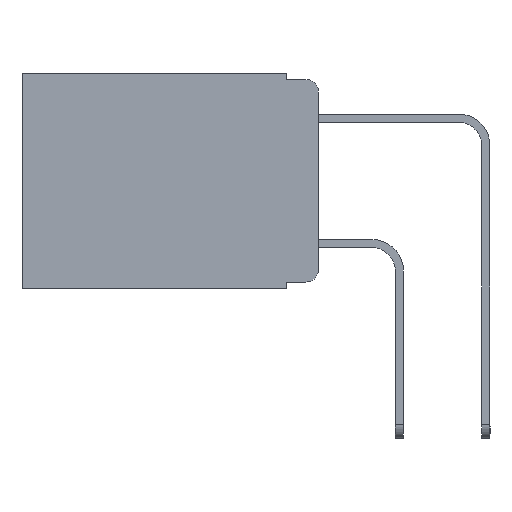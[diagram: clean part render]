
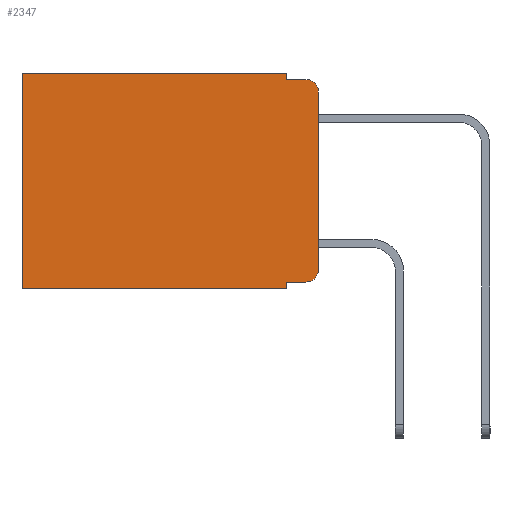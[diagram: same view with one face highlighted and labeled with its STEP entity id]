
A CAD part, left-side view. The second image highlights one B-rep face of the part: STEP entity #2347.
In plain terms, the highlighted planar face has unit normal (-1, 0, 0).
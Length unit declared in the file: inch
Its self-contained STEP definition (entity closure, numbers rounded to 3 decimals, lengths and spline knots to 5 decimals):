
#246 = EDGE_CURVE ( 'NONE', #7713, #7204, #11973, .T. ) ;
#724 = EDGE_CURVE ( 'NONE', #7204, #9671, #5408, .T. ) ;
#1034 = DIRECTION ( 'NONE',  ( 0., 0., -1. ) ) ;
#1077 = DIRECTION ( 'NONE',  ( -1., 0., 0. ) ) ;
#1807 = CARTESIAN_POINT ( 'NONE',  ( 0.298, 0.051, -0.343 ) ) ;
#1975 = VECTOR ( 'NONE', #14426, 39.37008 ) ;
#1977 = VECTOR ( 'NONE', #2763, 39.37008 ) ;
#2004 = ORIENTED_EDGE ( 'NONE', *, *, #11265, .T. ) ;
#2230 = DIRECTION ( 'NONE',  ( 0., 1., 0. ) ) ;
#2259 = CARTESIAN_POINT ( 'NONE',  ( 0.298, 0.051, 0. ) ) ;
#2347 = ADVANCED_FACE ( 'NONE', ( #16004 ), #14722, .F. ) ;
#2424 = LINE ( 'NONE', #2259, #12015 ) ;
#2763 = DIRECTION ( 'NONE',  ( 0., -1., 0. ) ) ;
#3219 = VERTEX_POINT ( 'NONE', #10655 ) ;
#3571 = ORIENTED_EDGE ( 'NONE', *, *, #6054, .T. ) ;
#3984 = CIRCLE ( 'NONE', #5084, 0.02 ) ;
#4034 = VECTOR ( 'NONE', #10815, 39.37008 ) ;
#4037 = VERTEX_POINT ( 'NONE', #16768 ) ;
#4116 = EDGE_CURVE ( 'NONE', #7650, #8345, #5388, .T. ) ;
#4186 = CARTESIAN_POINT ( 'NONE',  ( 0.298, 0., 0. ) ) ;
#4478 = CARTESIAN_POINT ( 'NONE',  ( 0.298, 0.02, -0.313 ) ) ;
#5084 = AXIS2_PLACEMENT_3D ( 'NONE', #5163, #1077, #13001 ) ;
#5163 = CARTESIAN_POINT ( 'NONE',  ( 0.298, 0.02, -0.03 ) ) ;
#5388 = LINE ( 'NONE', #6850, #5548 ) ;
#5408 = LINE ( 'NONE', #6866, #4034 ) ;
#5415 = CARTESIAN_POINT ( 'NONE',  ( 0.298, 0.02, -0.01 ) ) ;
#5548 = VECTOR ( 'NONE', #5563, 39.37008 ) ;
#5563 = DIRECTION ( 'NONE',  ( 0., 1., 0. ) ) ;
#5756 = EDGE_CURVE ( 'NONE', #16149, #7650, #2424, .T. ) ;
#5963 = LINE ( 'NONE', #14050, #16222 ) ;
#6054 = EDGE_CURVE ( 'NONE', #15632, #8345, #16400, .T. ) ;
#6850 = CARTESIAN_POINT ( 'NONE',  ( 0.298, 0., -0.343 ) ) ;
#6866 = CARTESIAN_POINT ( 'NONE',  ( 0.298, 0.051, -0.01 ) ) ;
#7204 = VERTEX_POINT ( 'NONE', #9839 ) ;
#7392 = DIRECTION ( 'NONE',  ( 0., 0., -1. ) ) ;
#7650 = VERTEX_POINT ( 'NONE', #1807 ) ;
#7713 = VERTEX_POINT ( 'NONE', #15015 ) ;
#7730 = CARTESIAN_POINT ( 'NONE',  ( 0.298, 0., 0. ) ) ;
#7798 = EDGE_CURVE ( 'NONE', #7713, #15632, #5963, .T. ) ;
#8127 = VECTOR ( 'NONE', #7392, 39.37008 ) ;
#8345 = VERTEX_POINT ( 'NONE', #14203 ) ;
#8360 = DIRECTION ( 'NONE',  ( 0., 0., -1. ) ) ;
#8661 = ORIENTED_EDGE ( 'NONE', *, *, #246, .F. ) ;
#9184 = DIRECTION ( 'NONE',  ( 1., 0., 0. ) ) ;
#9462 = ORIENTED_EDGE ( 'NONE', *, *, #724, .F. ) ;
#9671 = VERTEX_POINT ( 'NONE', #5415 ) ;
#9743 = DIRECTION ( 'NONE',  ( 0., 0., -1. ) ) ;
#9839 = CARTESIAN_POINT ( 'NONE',  ( 0.298, 0.051, -0.01 ) ) ;
#10168 = AXIS2_PLACEMENT_3D ( 'NONE', #4186, #9184, #10467 ) ;
#10467 = DIRECTION ( 'NONE',  ( 0., 0., -1. ) ) ;
#10603 = EDGE_CURVE ( 'NONE', #16149, #4037, #13464, .T. ) ;
#10655 = CARTESIAN_POINT ( 'NONE',  ( 0.298, 0., -0.03 ) ) ;
#10780 = CARTESIAN_POINT ( 'NONE',  ( 0.298, 0.051, -0.333 ) ) ;
#10815 = DIRECTION ( 'NONE',  ( 0., -1., 0. ) ) ;
#10861 = ORIENTED_EDGE ( 'NONE', *, *, #5756, .F. ) ;
#11265 = EDGE_CURVE ( 'NONE', #4037, #13107, #16872, .T. ) ;
#11491 = ORIENTED_EDGE ( 'NONE', *, *, #10603, .T. ) ;
#11973 = LINE ( 'NONE', #16928, #1975 ) ;
#12015 = VECTOR ( 'NONE', #1034, 39.37008 ) ;
#12155 = CARTESIAN_POINT ( 'NONE',  ( 0.298, 0.473, 0. ) ) ;
#12353 = ORIENTED_EDGE ( 'NONE', *, *, #7798, .T. ) ;
#12786 = ORIENTED_EDGE ( 'NONE', *, *, #14777, .T. ) ;
#12974 = CARTESIAN_POINT ( 'NONE',  ( 0.298, 0., -0.313 ) ) ;
#13001 = DIRECTION ( 'NONE',  ( 0., 0., -1. ) ) ;
#13107 = VERTEX_POINT ( 'NONE', #12974 ) ;
#13464 = LINE ( 'NONE', #10780, #1977 ) ;
#13752 = EDGE_LOOP ( 'NONE', ( #14237, #12786, #9462, #8661, #12353, #3571, #16796, #10861, #11491, #2004 ) ) ;
#13835 = AXIS2_PLACEMENT_3D ( 'NONE', #4478, #16204, #8360 ) ;
#13981 = CARTESIAN_POINT ( 'NONE',  ( 0.298, 0.051, -0.333 ) ) ;
#14050 = CARTESIAN_POINT ( 'NONE',  ( 0.298, 0., 0. ) ) ;
#14114 = LINE ( 'NONE', #7730, #8127 ) ;
#14203 = CARTESIAN_POINT ( 'NONE',  ( 0.298, 0.473, -0.343 ) ) ;
#14237 = ORIENTED_EDGE ( 'NONE', *, *, #15296, .F. ) ;
#14426 = DIRECTION ( 'NONE',  ( 0., 0., -1. ) ) ;
#14722 = PLANE ( 'NONE',  #10168 ) ;
#14777 = EDGE_CURVE ( 'NONE', #3219, #9671, #3984, .T. ) ;
#15015 = CARTESIAN_POINT ( 'NONE',  ( 0.298, 0.051, 0. ) ) ;
#15222 = CARTESIAN_POINT ( 'NONE',  ( 0.298, 0.473, 0. ) ) ;
#15296 = EDGE_CURVE ( 'NONE', #3219, #13107, #14114, .T. ) ;
#15632 = VERTEX_POINT ( 'NONE', #15222 ) ;
#16004 = FACE_OUTER_BOUND ( 'NONE', #13752, .T. ) ;
#16149 = VERTEX_POINT ( 'NONE', #13981 ) ;
#16204 = DIRECTION ( 'NONE',  ( -1., 0., 0. ) ) ;
#16222 = VECTOR ( 'NONE', #2230, 39.37008 ) ;
#16400 = LINE ( 'NONE', #12155, #16731 ) ;
#16731 = VECTOR ( 'NONE', #9743, 39.37008 ) ;
#16768 = CARTESIAN_POINT ( 'NONE',  ( 0.298, 0.02, -0.333 ) ) ;
#16796 = ORIENTED_EDGE ( 'NONE', *, *, #4116, .F. ) ;
#16872 = CIRCLE ( 'NONE', #13835, 0.02 ) ;
#16928 = CARTESIAN_POINT ( 'NONE',  ( 0.298, 0.051, 0. ) ) ;
